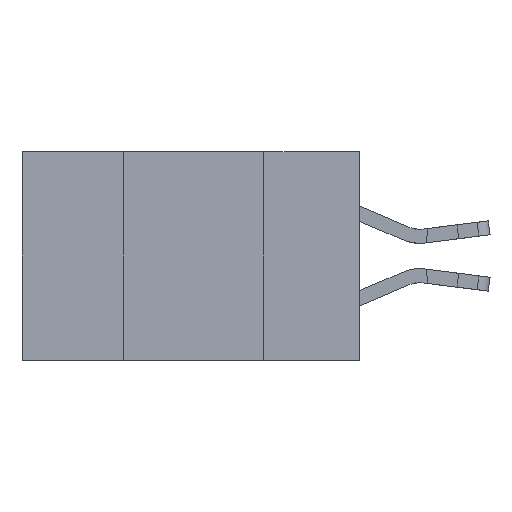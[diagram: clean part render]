
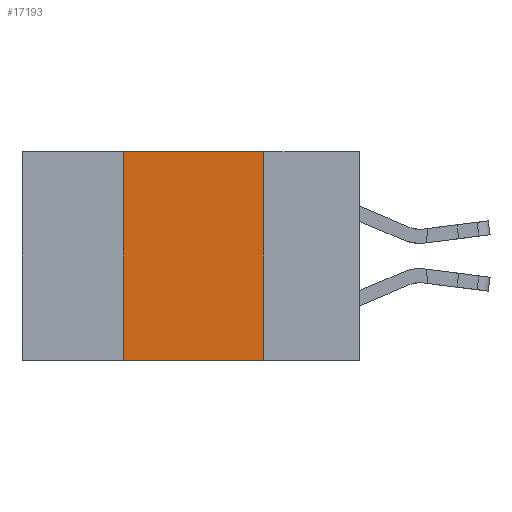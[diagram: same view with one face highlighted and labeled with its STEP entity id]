
A CAD part, left-side view. The second image highlights one B-rep face of the part: STEP entity #17193.
In plain terms, the highlighted planar face has unit normal (-1, 0, 0).
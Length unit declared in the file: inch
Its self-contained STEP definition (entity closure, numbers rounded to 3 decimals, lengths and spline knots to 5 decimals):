
#604 = CARTESIAN_POINT ( 'NONE',  ( 0., 0.6, -0.37 ) ) ;
#1040 = LINE ( 'NONE', #25518, #12360 ) ;
#1406 = ORIENTED_EDGE ( 'NONE', *, *, #15148, .F. ) ;
#1552 = EDGE_CURVE ( 'NONE', #7941, #22165, #1040, .T. ) ;
#1988 = DIRECTION ( 'NONE',  ( 0., -1., 0. ) ) ;
#2279 = ORIENTED_EDGE ( 'NONE', *, *, #9251, .F. ) ;
#4390 = CARTESIAN_POINT ( 'NONE',  ( 0., 0.42, 0. ) ) ;
#4595 = FACE_OUTER_BOUND ( 'NONE', #35696, .T. ) ;
#5083 = VECTOR ( 'NONE', #12987, 39.37008 ) ;
#5214 = LINE ( 'NONE', #9900, #19520 ) ;
#6240 = DIRECTION ( 'NONE',  ( 0., 0., -1. ) ) ;
#7251 = VERTEX_POINT ( 'NONE', #35865 ) ;
#7941 = VERTEX_POINT ( 'NONE', #21806 ) ;
#8865 = EDGE_CURVE ( 'NONE', #27517, #22165, #26822, .T. ) ;
#9251 = EDGE_CURVE ( 'NONE', #27517, #7251, #14616, .T. ) ;
#9900 = CARTESIAN_POINT ( 'NONE',  ( 0., 0.6, 0. ) ) ;
#10134 = PLANE ( 'NONE',  #14999 ) ;
#11642 = VECTOR ( 'NONE', #22937, 39.37008 ) ;
#12360 = VECTOR ( 'NONE', #6240, 39.37008 ) ;
#12987 = DIRECTION ( 'NONE',  ( 0., 0., 1. ) ) ;
#14616 = LINE ( 'NONE', #4390, #5083 ) ;
#14694 = CARTESIAN_POINT ( 'NONE',  ( 0., 0.42, -0.37 ) ) ;
#14999 = AXIS2_PLACEMENT_3D ( 'NONE', #32751, #32492, #35173 ) ;
#15148 = EDGE_CURVE ( 'NONE', #7251, #7941, #5214, .T. ) ;
#17193 = ADVANCED_FACE ( 'NONE', ( #4595 ), #10134, .F. ) ;
#17642 = CARTESIAN_POINT ( 'NONE',  ( 0., 0.17, -0.37 ) ) ;
#17738 = ORIENTED_EDGE ( 'NONE', *, *, #1552, .F. ) ;
#18622 = ORIENTED_EDGE ( 'NONE', *, *, #8865, .T. ) ;
#19520 = VECTOR ( 'NONE', #1988, 39.37008 ) ;
#21806 = CARTESIAN_POINT ( 'NONE',  ( 0., 0.17, 0. ) ) ;
#22165 = VERTEX_POINT ( 'NONE', #17642 ) ;
#22937 = DIRECTION ( 'NONE',  ( 0., -1., 0. ) ) ;
#25518 = CARTESIAN_POINT ( 'NONE',  ( 0., 0.17, 0. ) ) ;
#26822 = LINE ( 'NONE', #604, #11642 ) ;
#27517 = VERTEX_POINT ( 'NONE', #14694 ) ;
#32492 = DIRECTION ( 'NONE',  ( 1., 0., 0. ) ) ;
#32751 = CARTESIAN_POINT ( 'NONE',  ( 0., 0.6, 0. ) ) ;
#35173 = DIRECTION ( 'NONE',  ( 0., 0., -1. ) ) ;
#35696 = EDGE_LOOP ( 'NONE', ( #17738, #1406, #2279, #18622 ) ) ;
#35865 = CARTESIAN_POINT ( 'NONE',  ( 0., 0.42, 0. ) ) ;
